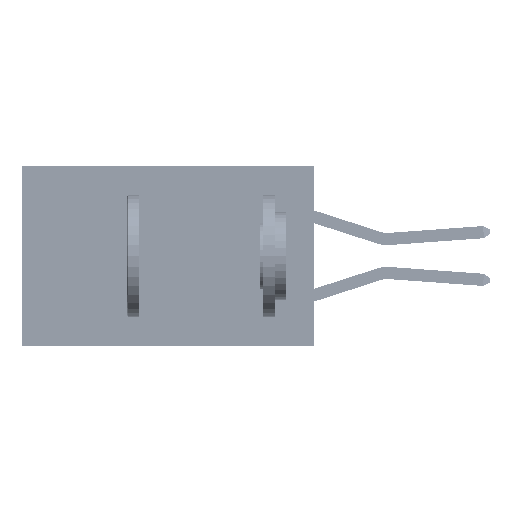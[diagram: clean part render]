
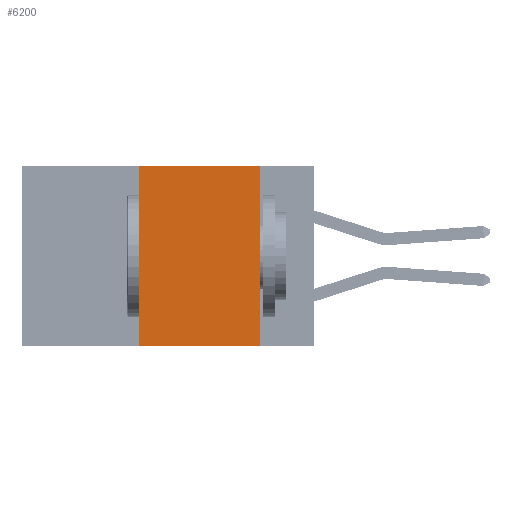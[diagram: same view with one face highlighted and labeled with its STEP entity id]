
A CAD part, left-side view. The second image highlights one B-rep face of the part: STEP entity #6200.
In plain terms, the highlighted planar face has unit normal (-1, 0, 0).
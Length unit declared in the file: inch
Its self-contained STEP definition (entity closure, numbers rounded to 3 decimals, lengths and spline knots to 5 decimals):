
#1439 = ORIENTED_EDGE ( 'NONE', *, *, #11755, .F. ) ;
#2129 = DIRECTION ( 'NONE',  ( 0., 0., 1. ) ) ;
#5217 = EDGE_CURVE ( 'NONE', #47752, #30083, #12192, .T. ) ;
#5712 = ORIENTED_EDGE ( 'NONE', *, *, #30749, .F. ) ;
#6200 = ADVANCED_FACE ( 'NONE', ( #19816 ), #52603, .F. ) ;
#6430 = CARTESIAN_POINT ( 'NONE',  ( 0., 0.11, 0. ) ) ;
#7409 = ORIENTED_EDGE ( 'NONE', *, *, #44606, .F. ) ;
#9326 = CARTESIAN_POINT ( 'NONE',  ( 0., 0.6, -0.37 ) ) ;
#10443 = VECTOR ( 'NONE', #2129, 39.37008 ) ;
#11093 = LINE ( 'NONE', #23078, #10443 ) ;
#11755 = EDGE_CURVE ( 'NONE', #24392, #30083, #21250, .T. ) ;
#11840 = LINE ( 'NONE', #20711, #43405 ) ;
#12192 = LINE ( 'NONE', #9326, #50836 ) ;
#15883 = CARTESIAN_POINT ( 'NONE',  ( 0., 0.6, 0. ) ) ;
#16856 = CARTESIAN_POINT ( 'NONE',  ( 0., 0.36, 0. ) ) ;
#19816 = FACE_OUTER_BOUND ( 'NONE', #22048, .T. ) ;
#20711 = CARTESIAN_POINT ( 'NONE',  ( 0., 0.6, 0. ) ) ;
#21250 = LINE ( 'NONE', #6430, #31555 ) ;
#22048 = EDGE_LOOP ( 'NONE', ( #1439, #5712, #7409, #27757 ) ) ;
#23078 = CARTESIAN_POINT ( 'NONE',  ( 0., 0.36, 0. ) ) ;
#23289 = AXIS2_PLACEMENT_3D ( 'NONE', #15883, #24211, #32253 ) ;
#24211 = DIRECTION ( 'NONE',  ( 1., 0., 0. ) ) ;
#24392 = VERTEX_POINT ( 'NONE', #51173 ) ;
#27757 = ORIENTED_EDGE ( 'NONE', *, *, #5217, .T. ) ;
#30083 = VERTEX_POINT ( 'NONE', #48782 ) ;
#30749 = EDGE_CURVE ( 'NONE', #50167, #24392, #11840, .T. ) ;
#31555 = VECTOR ( 'NONE', #35175, 39.37008 ) ;
#32253 = DIRECTION ( 'NONE',  ( 0., 0., -1. ) ) ;
#32279 = CARTESIAN_POINT ( 'NONE',  ( 0., 0.36, -0.37 ) ) ;
#34485 = DIRECTION ( 'NONE',  ( 0., -1., 0. ) ) ;
#35175 = DIRECTION ( 'NONE',  ( 0., 0., -1. ) ) ;
#43405 = VECTOR ( 'NONE', #49442, 39.37008 ) ;
#44606 = EDGE_CURVE ( 'NONE', #47752, #50167, #11093, .T. ) ;
#47752 = VERTEX_POINT ( 'NONE', #32279 ) ;
#48782 = CARTESIAN_POINT ( 'NONE',  ( 0., 0.11, -0.37 ) ) ;
#49442 = DIRECTION ( 'NONE',  ( 0., -1., 0. ) ) ;
#50167 = VERTEX_POINT ( 'NONE', #16856 ) ;
#50836 = VECTOR ( 'NONE', #34485, 39.37008 ) ;
#51173 = CARTESIAN_POINT ( 'NONE',  ( 0., 0.11, 0. ) ) ;
#52603 = PLANE ( 'NONE',  #23289 ) ;
